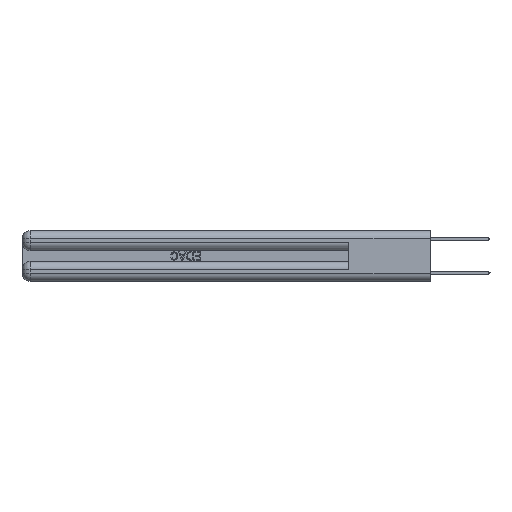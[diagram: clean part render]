
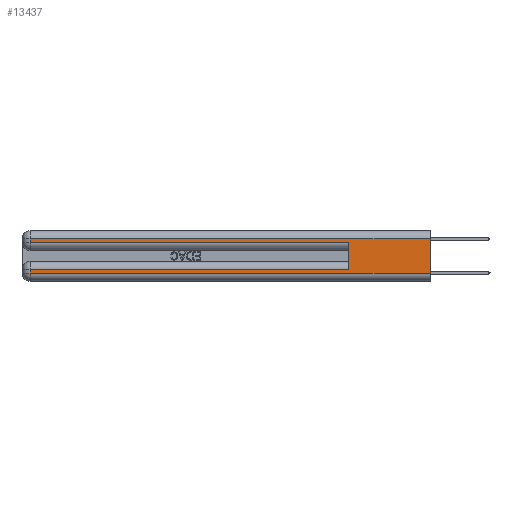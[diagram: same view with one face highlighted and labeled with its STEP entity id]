
A CAD part, left-side view. The second image highlights one B-rep face of the part: STEP entity #13437.
In plain terms, the highlighted planar face has unit normal (-1, 0, 0).
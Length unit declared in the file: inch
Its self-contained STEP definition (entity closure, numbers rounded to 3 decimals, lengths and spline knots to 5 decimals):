
#1631 = VECTOR ( 'NONE', #9969, 39.37008 ) ;
#1853 = ORIENTED_EDGE ( 'NONE', *, *, #18007, .F. ) ;
#2151 = CARTESIAN_POINT ( 'NONE',  ( 0., 0., 0.06 ) ) ;
#2995 = VERTEX_POINT ( 'NONE', #19575 ) ;
#3194 = ORIENTED_EDGE ( 'NONE', *, *, #23758, .T. ) ;
#4016 = DIRECTION ( 'NONE',  ( 1., 0., 0. ) ) ;
#5278 = LINE ( 'NONE', #36541, #36009 ) ;
#6543 = CARTESIAN_POINT ( 'NONE',  ( 0., 2.94, 0.37 ) ) ;
#6690 = VECTOR ( 'NONE', #30090, 39.37008 ) ;
#6869 = VERTEX_POINT ( 'NONE', #35450 ) ;
#7202 = FACE_OUTER_BOUND ( 'NONE', #10866, .T. ) ;
#7642 = LINE ( 'NONE', #32911, #9684 ) ;
#7896 = DIRECTION ( 'NONE',  ( 0., 0., -1. ) ) ;
#7921 = DIRECTION ( 'NONE',  ( 0., -1., 0. ) ) ;
#8617 = DIRECTION ( 'NONE',  ( 0., 1., 0. ) ) ;
#9684 = VECTOR ( 'NONE', #18592, 39.37008 ) ;
#9900 = EDGE_CURVE ( 'NONE', #19729, #35794, #26386, .T. ) ;
#9969 = DIRECTION ( 'NONE',  ( 0., 0., -1. ) ) ;
#10113 = ORIENTED_EDGE ( 'NONE', *, *, #15265, .T. ) ;
#10183 = ORIENTED_EDGE ( 'NONE', *, *, #9900, .T. ) ;
#10620 = DIRECTION ( 'NONE',  ( 0., -1., 0. ) ) ;
#10788 = ORIENTED_EDGE ( 'NONE', *, *, #27623, .T. ) ;
#10866 = EDGE_LOOP ( 'NONE', ( #25290, #10788, #25057, #10113, #1853, #10183, #3194, #36790 ) ) ;
#11271 = EDGE_CURVE ( 'NONE', #13349, #6869, #26933, .T. ) ;
#11641 = CARTESIAN_POINT ( 'NONE',  ( 0., 0., 0.31 ) ) ;
#11695 = CARTESIAN_POINT ( 'NONE',  ( 0., 0., 0.085 ) ) ;
#12772 = LINE ( 'NONE', #6543, #6690 ) ;
#13321 = VECTOR ( 'NONE', #10620, 39.37008 ) ;
#13349 = VERTEX_POINT ( 'NONE', #31627 ) ;
#13437 = ADVANCED_FACE ( 'NONE', ( #7202 ), #30206, .F. ) ;
#15265 = EDGE_CURVE ( 'NONE', #37145, #35077, #5278, .T. ) ;
#15507 = DIRECTION ( 'NONE',  ( 0., 0., -1. ) ) ;
#18007 = EDGE_CURVE ( 'NONE', #19729, #35077, #7642, .T. ) ;
#18252 = VERTEX_POINT ( 'NONE', #28561 ) ;
#18336 = CARTESIAN_POINT ( 'NONE',  ( 0., 0., 0.37 ) ) ;
#18592 = DIRECTION ( 'NONE',  ( 0., 0., 1. ) ) ;
#18638 = EDGE_CURVE ( 'NONE', #2995, #6869, #31165, .T. ) ;
#19204 = CARTESIAN_POINT ( 'NONE',  ( 0., 2.94, 0.37 ) ) ;
#19575 = CARTESIAN_POINT ( 'NONE',  ( 0., 2.94, 0.06 ) ) ;
#19729 = VERTEX_POINT ( 'NONE', #32010 ) ;
#20927 = EDGE_CURVE ( 'NONE', #18252, #37145, #33901, .T. ) ;
#23742 = DIRECTION ( 'NONE',  ( 0., 1., 0. ) ) ;
#23758 = EDGE_CURVE ( 'NONE', #35794, #2995, #12772, .T. ) ;
#25057 = ORIENTED_EDGE ( 'NONE', *, *, #20927, .T. ) ;
#25290 = ORIENTED_EDGE ( 'NONE', *, *, #11271, .F. ) ;
#25951 = LINE ( 'NONE', #11641, #32762 ) ;
#26386 = LINE ( 'NONE', #11695, #29270 ) ;
#26933 = LINE ( 'NONE', #36144, #1631 ) ;
#27623 = EDGE_CURVE ( 'NONE', #13349, #18252, #25951, .T. ) ;
#28561 = CARTESIAN_POINT ( 'NONE',  ( 0., 2.94, 0.31 ) ) ;
#28904 = VECTOR ( 'NONE', #7896, 39.37008 ) ;
#29270 = VECTOR ( 'NONE', #23742, 39.37008 ) ;
#30090 = DIRECTION ( 'NONE',  ( 0., 0., -1. ) ) ;
#30206 = PLANE ( 'NONE',  #33047 ) ;
#30491 = CARTESIAN_POINT ( 'NONE',  ( 0., 2.94, 0.085 ) ) ;
#31165 = LINE ( 'NONE', #2151, #13321 ) ;
#31627 = CARTESIAN_POINT ( 'NONE',  ( 0., 0., 0.31 ) ) ;
#32010 = CARTESIAN_POINT ( 'NONE',  ( 0., 0.6, 0.085 ) ) ;
#32762 = VECTOR ( 'NONE', #8617, 39.37008 ) ;
#32911 = CARTESIAN_POINT ( 'NONE',  ( 0., 0.6, 0.145 ) ) ;
#33047 = AXIS2_PLACEMENT_3D ( 'NONE', #18336, #4016, #15507 ) ;
#33784 = CARTESIAN_POINT ( 'NONE',  ( 0., 0.6, 0.285 ) ) ;
#33901 = LINE ( 'NONE', #19204, #28904 ) ;
#34998 = CARTESIAN_POINT ( 'NONE',  ( 0., 2.94, 0.285 ) ) ;
#35077 = VERTEX_POINT ( 'NONE', #33784 ) ;
#35450 = CARTESIAN_POINT ( 'NONE',  ( 0., 0., 0.06 ) ) ;
#35794 = VERTEX_POINT ( 'NONE', #30491 ) ;
#36009 = VECTOR ( 'NONE', #7921, 39.37008 ) ;
#36144 = CARTESIAN_POINT ( 'NONE',  ( 0., 0., 0.37 ) ) ;
#36541 = CARTESIAN_POINT ( 'NONE',  ( 0., 0., 0.285 ) ) ;
#36790 = ORIENTED_EDGE ( 'NONE', *, *, #18638, .T. ) ;
#37145 = VERTEX_POINT ( 'NONE', #34998 ) ;
